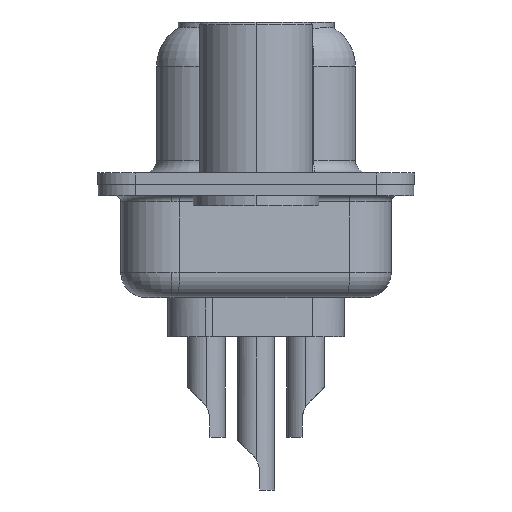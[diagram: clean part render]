
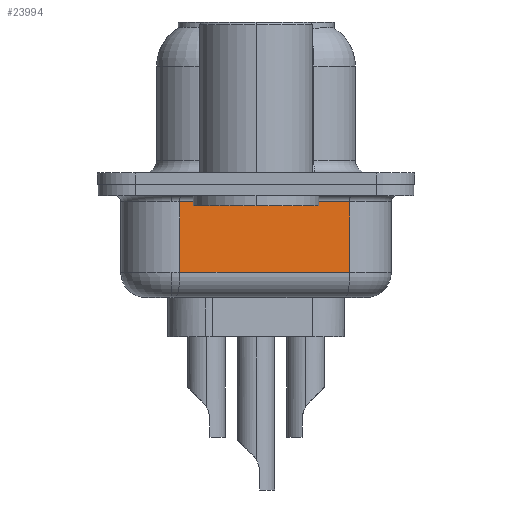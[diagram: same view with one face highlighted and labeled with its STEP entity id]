
A CAD part, left-side view. The second image highlights one B-rep face of the part: STEP entity #23994.
In plain terms, the highlighted planar face has unit normal (-0.985, -0.174, 0).
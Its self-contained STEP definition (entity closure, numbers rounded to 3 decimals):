
#291 = AXIS2_PLACEMENT_3D ( 'NONE', #4067, #22446, #8137 ) ;
#564 = CARTESIAN_POINT ( 'NONE',  ( 2.84, 3.028, -4.5 ) ) ;
#1044 = VERTEX_POINT ( 'NONE', #22892 ) ;
#4067 = CARTESIAN_POINT ( 'NONE',  ( 2.84, 3.028, -4.5 ) ) ;
#4850 = LINE ( 'NONE', #14065, #11504 ) ;
#5584 = EDGE_CURVE ( 'NONE', #1044, #26214, #10302, .T. ) ;
#6038 = VERTEX_POINT ( 'NONE', #24418 ) ;
#7521 = VECTOR ( 'NONE', #12616, 1000. ) ;
#8137 = DIRECTION ( 'NONE',  ( -0.174, 0.985, 0. ) ) ;
#10037 = ORIENTED_EDGE ( 'NONE', *, *, #28762, .F. ) ;
#10082 = VECTOR ( 'NONE', #22815, 1000. ) ;
#10302 = LINE ( 'NONE', #10608, #19611 ) ;
#10608 = CARTESIAN_POINT ( 'NONE',  ( 4.031, -3.722, -4.5 ) ) ;
#11504 = VECTOR ( 'NONE', #18867, 1000. ) ;
#12548 = EDGE_CURVE ( 'NONE', #26214, #16202, #4850, .T. ) ;
#12616 = DIRECTION ( 'NONE',  ( 0., 0., 1. ) ) ;
#12969 = PLANE ( 'NONE',  #291 ) ;
#14065 = CARTESIAN_POINT ( 'NONE',  ( 2.84, 3.028, -0.7 ) ) ;
#14432 = LINE ( 'NONE', #564, #7521 ) ;
#15190 = ORIENTED_EDGE ( 'NONE', *, *, #15348, .T. ) ;
#15348 = EDGE_CURVE ( 'NONE', #6038, #1044, #27935, .T. ) ;
#16202 = VERTEX_POINT ( 'NONE', #19374 ) ;
#17684 = DIRECTION ( 'NONE',  ( 0., 0., 1. ) ) ;
#18867 = DIRECTION ( 'NONE',  ( -0.174, 0.985, 0. ) ) ;
#19374 = CARTESIAN_POINT ( 'NONE',  ( 2.84, 3.028, -0.7 ) ) ;
#19611 = VECTOR ( 'NONE', #17684, 1000. ) ;
#19661 = ORIENTED_EDGE ( 'NONE', *, *, #5584, .T. ) ;
#20708 = CARTESIAN_POINT ( 'NONE',  ( 2.84, 3.028, -3.5 ) ) ;
#20843 = CARTESIAN_POINT ( 'NONE',  ( 4.031, -3.722, -0.7 ) ) ;
#22331 = EDGE_LOOP ( 'NONE', ( #10037, #15190, #19661, #22706 ) ) ;
#22446 = DIRECTION ( 'NONE',  ( 0.985, 0.174, 0. ) ) ;
#22706 = ORIENTED_EDGE ( 'NONE', *, *, #12548, .T. ) ;
#22815 = DIRECTION ( 'NONE',  ( 0.174, -0.985, 0. ) ) ;
#22892 = CARTESIAN_POINT ( 'NONE',  ( 4.031, -3.722, -3.5 ) ) ;
#23994 = ADVANCED_FACE ( 'NONE', ( #28781 ), #12969, .F. ) ;
#24418 = CARTESIAN_POINT ( 'NONE',  ( 2.84, 3.028, -3.5 ) ) ;
#26214 = VERTEX_POINT ( 'NONE', #20843 ) ;
#27935 = LINE ( 'NONE', #20708, #10082 ) ;
#28762 = EDGE_CURVE ( 'NONE', #6038, #16202, #14432, .T. ) ;
#28781 = FACE_OUTER_BOUND ( 'NONE', #22331, .T. ) ;
